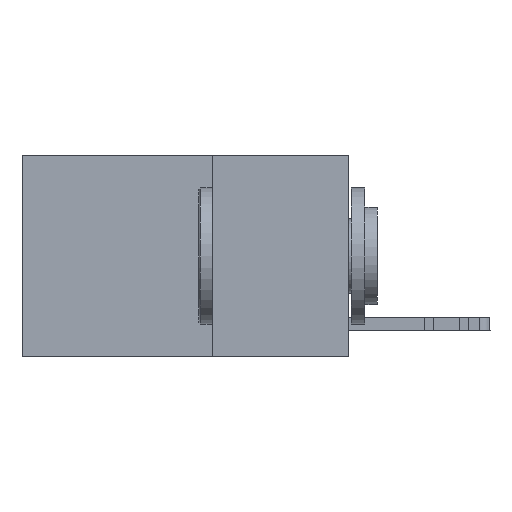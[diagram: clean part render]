
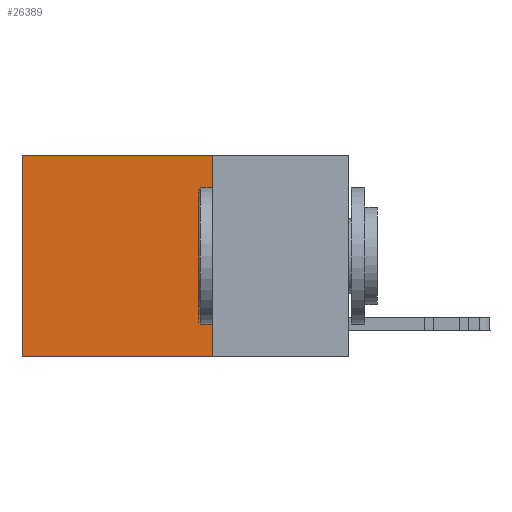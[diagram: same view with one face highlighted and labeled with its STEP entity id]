
A CAD part, left-side view. The second image highlights one B-rep face of the part: STEP entity #26389.
In plain terms, the highlighted planar face has unit normal (-1, 0, 0).
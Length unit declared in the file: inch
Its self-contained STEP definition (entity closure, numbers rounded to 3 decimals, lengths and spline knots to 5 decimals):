
#1268 = ORIENTED_EDGE ( 'NONE', *, *, #16543, .F. ) ;
#2039 = DIRECTION ( 'NONE',  ( 0., 1., 0. ) ) ;
#2192 = DIRECTION ( 'NONE',  ( 0., 0., -1. ) ) ;
#4036 = LINE ( 'NONE', #12536, #23248 ) ;
#4382 = DIRECTION ( 'NONE',  ( 0., 0., -1. ) ) ;
#4635 = CARTESIAN_POINT ( 'NONE',  ( 0.2625, 0.6, -0.37 ) ) ;
#4773 = CARTESIAN_POINT ( 'NONE',  ( 0.2625, 0.6, 0. ) ) ;
#5707 = EDGE_CURVE ( 'NONE', #14545, #18206, #26244, .T. ) ;
#6170 = EDGE_CURVE ( 'NONE', #13497, #13330, #17546, .T. ) ;
#6784 = CARTESIAN_POINT ( 'NONE',  ( 0.2625, 0.25, 0. ) ) ;
#8133 = ORIENTED_EDGE ( 'NONE', *, *, #9404, .T. ) ;
#8298 = LINE ( 'NONE', #23777, #23471 ) ;
#9404 = EDGE_CURVE ( 'NONE', #14545, #13497, #8298, .T. ) ;
#11144 = VECTOR ( 'NONE', #26066, 39.37008 ) ;
#12310 = ORIENTED_EDGE ( 'NONE', *, *, #6170, .T. ) ;
#12536 = CARTESIAN_POINT ( 'NONE',  ( 0.2625, 0.25, -0.37 ) ) ;
#13115 = DIRECTION ( 'NONE',  ( 1., 0., 0. ) ) ;
#13330 = VERTEX_POINT ( 'NONE', #4635 ) ;
#13497 = VERTEX_POINT ( 'NONE', #4773 ) ;
#14545 = VERTEX_POINT ( 'NONE', #16438 ) ;
#14931 = CARTESIAN_POINT ( 'NONE',  ( 0.2625, 0.25, -0.37 ) ) ;
#16438 = CARTESIAN_POINT ( 'NONE',  ( 0.2625, 0.25, 0. ) ) ;
#16543 = EDGE_CURVE ( 'NONE', #18206, #13330, #4036, .T. ) ;
#17253 = DIRECTION ( 'NONE',  ( 0., 1., 0. ) ) ;
#17399 = CARTESIAN_POINT ( 'NONE',  ( 0.2625, 0.25, 0. ) ) ;
#17546 = LINE ( 'NONE', #24089, #11144 ) ;
#18206 = VERTEX_POINT ( 'NONE', #14931 ) ;
#19001 = VECTOR ( 'NONE', #4382, 39.37008 ) ;
#19826 = ORIENTED_EDGE ( 'NONE', *, *, #5707, .F. ) ;
#21646 = PLANE ( 'NONE',  #23507 ) ;
#23248 = VECTOR ( 'NONE', #2039, 39.37008 ) ;
#23471 = VECTOR ( 'NONE', #17253, 39.37008 ) ;
#23507 = AXIS2_PLACEMENT_3D ( 'NONE', #17399, #13115, #2192 ) ;
#23777 = CARTESIAN_POINT ( 'NONE',  ( 0.2625, 0.25, 0. ) ) ;
#24089 = CARTESIAN_POINT ( 'NONE',  ( 0.2625, 0.6, 0. ) ) ;
#26066 = DIRECTION ( 'NONE',  ( 0., 0., -1. ) ) ;
#26244 = LINE ( 'NONE', #6784, #19001 ) ;
#26279 = EDGE_LOOP ( 'NONE', ( #12310, #1268, #19826, #8133 ) ) ;
#26338 = FACE_OUTER_BOUND ( 'NONE', #26279, .T. ) ;
#26389 = ADVANCED_FACE ( 'NONE', ( #26338 ), #21646, .F. ) ;
